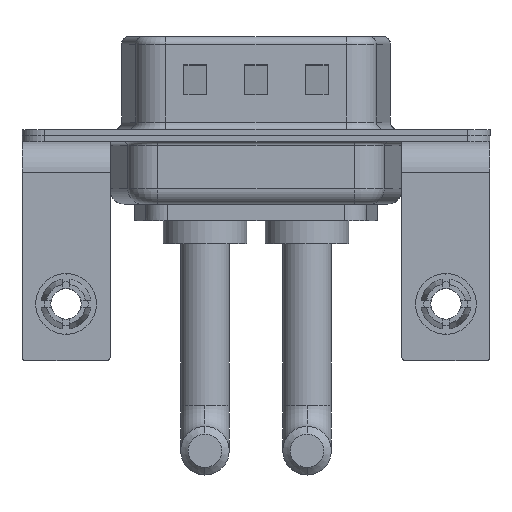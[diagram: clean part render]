
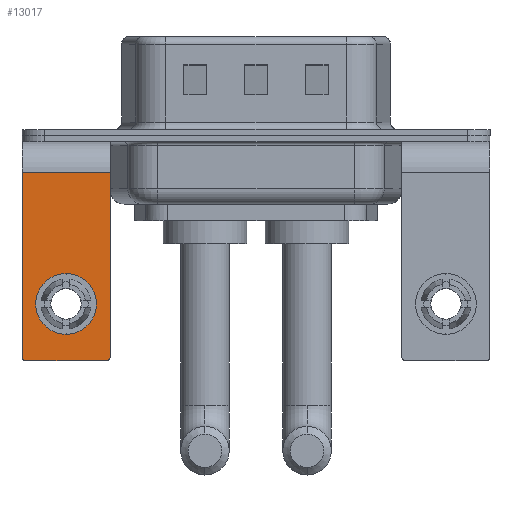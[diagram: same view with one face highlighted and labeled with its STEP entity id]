
A CAD part, front view. The second image highlights one B-rep face of the part: STEP entity #13017.
In plain terms, the highlighted planar face has unit normal (0, -1, 0).
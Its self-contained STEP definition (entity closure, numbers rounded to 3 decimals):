
#395 = CARTESIAN_POINT ( 'NONE',  ( -2.9, -6.25, -2.4 ) ) ;
#458 = AXIS2_PLACEMENT_3D ( 'NONE', #6104, #3215, #5930 ) ;
#619 = CARTESIAN_POINT ( 'NONE',  ( 2.9, -6.25, -14.8 ) ) ;
#802 = VERTEX_POINT ( 'NONE', #2307 ) ;
#1064 = DIRECTION ( 'NONE',  ( 0., 1., 0. ) ) ;
#1100 = DIRECTION ( 'NONE',  ( 0., -1., 0. ) ) ;
#1156 = VECTOR ( 'NONE', #9213, 1000. ) ;
#1391 = LINE ( 'NONE', #619, #4274 ) ;
#1562 = CIRCLE ( 'NONE', #458, 2. ) ;
#1867 = DIRECTION ( 'NONE',  ( 0., 0., 1. ) ) ;
#2307 = CARTESIAN_POINT ( 'NONE',  ( 2.9, -6.25, -14.55 ) ) ;
#2352 = PLANE ( 'NONE',  #7510 ) ;
#3215 = DIRECTION ( 'NONE',  ( 0., 1., 0. ) ) ;
#3444 = ORIENTED_EDGE ( 'NONE', *, *, #13616, .F. ) ;
#3804 = CARTESIAN_POINT ( 'NONE',  ( -2.9, -6.25, -2.4 ) ) ;
#4274 = VECTOR ( 'NONE', #11968, 1000. ) ;
#5245 = CARTESIAN_POINT ( 'NONE',  ( 0., -6.25, -11.07 ) ) ;
#5327 = LINE ( 'NONE', #395, #1156 ) ;
#5338 = EDGE_CURVE ( 'NONE', #12351, #7629, #15000, .T. ) ;
#5389 = CARTESIAN_POINT ( 'NONE',  ( -2.65, -6.25, -14.8 ) ) ;
#5930 = DIRECTION ( 'NONE',  ( 0., 0., 1. ) ) ;
#5970 = CARTESIAN_POINT ( 'NONE',  ( 2.9, -6.25, -2.4 ) ) ;
#6104 = CARTESIAN_POINT ( 'NONE',  ( 0., -6.25, -11.07 ) ) ;
#6247 = DIRECTION ( 'NONE',  ( 0., 0., 1. ) ) ;
#6418 = VERTEX_POINT ( 'NONE', #11533 ) ;
#6726 = LINE ( 'NONE', #13053, #7795 ) ;
#6885 = VERTEX_POINT ( 'NONE', #9590 ) ;
#7047 = CARTESIAN_POINT ( 'NONE',  ( 2.65, -6.25, -14.8 ) ) ;
#7200 = EDGE_CURVE ( 'NONE', #14844, #12351, #5327, .T. ) ;
#7214 = EDGE_CURVE ( 'NONE', #6885, #13060, #16310, .T. ) ;
#7510 = AXIS2_PLACEMENT_3D ( 'NONE', #7511, #1064, #6247 ) ;
#7511 = CARTESIAN_POINT ( 'NONE',  ( 2.9, -6.25, -2.4 ) ) ;
#7571 = DIRECTION ( 'NONE',  ( -1., 0., 0. ) ) ;
#7629 = VERTEX_POINT ( 'NONE', #5389 ) ;
#7630 = CARTESIAN_POINT ( 'NONE',  ( 0., -6.25, -9.07 ) ) ;
#7722 = AXIS2_PLACEMENT_3D ( 'NONE', #9565, #11188, #1867 ) ;
#7795 = VECTOR ( 'NONE', #11556, 1000. ) ;
#7800 = ORIENTED_EDGE ( 'NONE', *, *, #13150, .T. ) ;
#8759 = ORIENTED_EDGE ( 'NONE', *, *, #7200, .T. ) ;
#8780 = FACE_BOUND ( 'NONE', #13437, .T. ) ;
#9213 = DIRECTION ( 'NONE',  ( 0., 0., -1. ) ) ;
#9261 = ORIENTED_EDGE ( 'NONE', *, *, #14706, .T. ) ;
#9565 = CARTESIAN_POINT ( 'NONE',  ( -2.65, -6.25, -14.55 ) ) ;
#9590 = CARTESIAN_POINT ( 'NONE',  ( 0., -6.25, -13.07 ) ) ;
#10234 = VECTOR ( 'NONE', #7571, 1000. ) ;
#10246 = DIRECTION ( 'NONE',  ( 0., 0., 1. ) ) ;
#10563 = ORIENTED_EDGE ( 'NONE', *, *, #7214, .T. ) ;
#10637 = EDGE_LOOP ( 'NONE', ( #8759, #13135, #3444, #7800, #14797, #12338 ) ) ;
#11188 = DIRECTION ( 'NONE',  ( 0., -1., 0. ) ) ;
#11303 = LINE ( 'NONE', #5970, #10234 ) ;
#11325 = FACE_OUTER_BOUND ( 'NONE', #10637, .T. ) ;
#11533 = CARTESIAN_POINT ( 'NONE',  ( 2.9, -6.25, -2.4 ) ) ;
#11556 = DIRECTION ( 'NONE',  ( 0., 0., -1. ) ) ;
#11968 = DIRECTION ( 'NONE',  ( -1., 0., 0. ) ) ;
#12234 = CARTESIAN_POINT ( 'NONE',  ( -2.9, -6.25, -14.55 ) ) ;
#12338 = ORIENTED_EDGE ( 'NONE', *, *, #13909, .T. ) ;
#12351 = VERTEX_POINT ( 'NONE', #12234 ) ;
#12688 = CARTESIAN_POINT ( 'NONE',  ( 2.65, -6.25, -14.55 ) ) ;
#13017 = ADVANCED_FACE ( 'NONE', ( #8780, #11325 ), #2352, .F. ) ;
#13053 = CARTESIAN_POINT ( 'NONE',  ( 2.9, -6.25, -2.4 ) ) ;
#13060 = VERTEX_POINT ( 'NONE', #7630 ) ;
#13135 = ORIENTED_EDGE ( 'NONE', *, *, #5338, .T. ) ;
#13150 = EDGE_CURVE ( 'NONE', #15439, #802, #15614, .T. ) ;
#13259 = DIRECTION ( 'NONE',  ( 0., 1., 0. ) ) ;
#13317 = AXIS2_PLACEMENT_3D ( 'NONE', #5245, #13259, #14273 ) ;
#13437 = EDGE_LOOP ( 'NONE', ( #10563, #9261 ) ) ;
#13478 = EDGE_CURVE ( 'NONE', #6418, #802, #6726, .T. ) ;
#13616 = EDGE_CURVE ( 'NONE', #15439, #7629, #1391, .T. ) ;
#13909 = EDGE_CURVE ( 'NONE', #6418, #14844, #11303, .T. ) ;
#14273 = DIRECTION ( 'NONE',  ( 0., 0., 1. ) ) ;
#14706 = EDGE_CURVE ( 'NONE', #13060, #6885, #1562, .T. ) ;
#14788 = AXIS2_PLACEMENT_3D ( 'NONE', #12688, #1100, #10246 ) ;
#14797 = ORIENTED_EDGE ( 'NONE', *, *, #13478, .F. ) ;
#14844 = VERTEX_POINT ( 'NONE', #3804 ) ;
#15000 = CIRCLE ( 'NONE', #7722, 0.25 ) ;
#15439 = VERTEX_POINT ( 'NONE', #7047 ) ;
#15614 = CIRCLE ( 'NONE', #14788, 0.25 ) ;
#16310 = CIRCLE ( 'NONE', #13317, 2. ) ;
